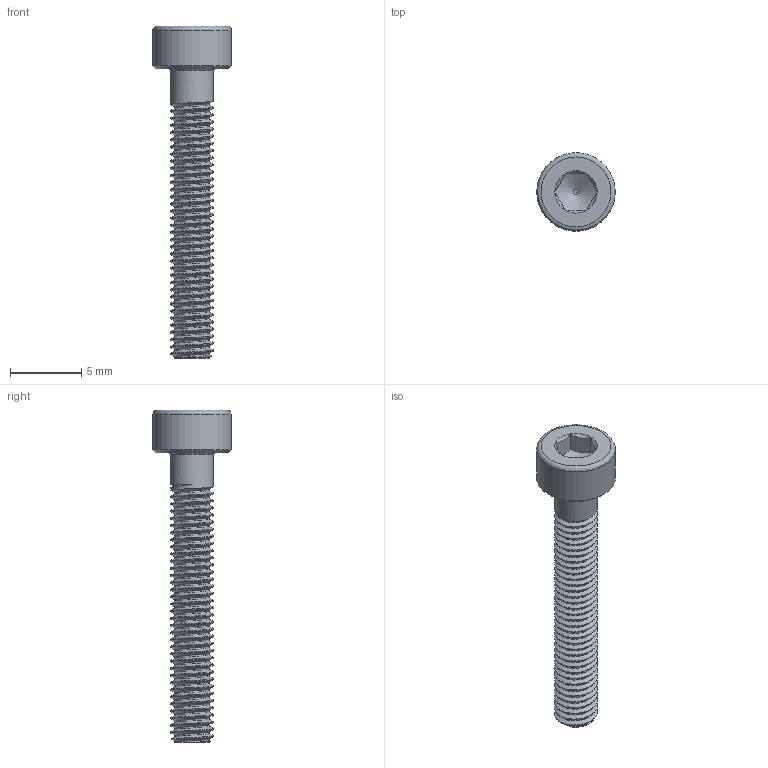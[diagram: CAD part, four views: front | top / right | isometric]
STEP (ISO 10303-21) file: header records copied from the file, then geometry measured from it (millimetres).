
FILE_DESCRIPTION(('FreeCAD Model'),'2;1');
FILE_NAME('Open CASCADE Shape Model','2022-12-07T11:22:07',('Author'),( ''),'Open CASCADE STEP processor 7.6','FreeCAD','Unknown');
FILE_SCHEMA(('AUTOMOTIVE_DESIGN { 1 0 10303 214 1 1 1 1 }'));
Length unit declared in the file: millimetre
Products named in the file (1): M3x20-Screw004
Bounding box: 5.5 x 5.5 x 23.25 mm (x, y, z)
Volume: 179.4 mm3; surface area: 381 mm2
Topology: 1 solids, 1 shells, 165 faces, 410 edges, 247 vertices
Faces by surface type: bspline 111, cylinder 37, plane 9, cone 5, revolution 2, sphere 1
Full cylindrical faces by diameter (mm): 3 x35, 5.5 x1
Entity records: 33886 total; most frequent: CARTESIAN_POINT 27625, ORIENTED_EDGE 816, PCURVE 816, DEFINITIONAL_REPRESENTATION 816, B_SPLINE_CURVE_WITH_KNOTS 759, DIRECTION 519, EDGE_CURVE 408, SURFACE_CURVE 400
